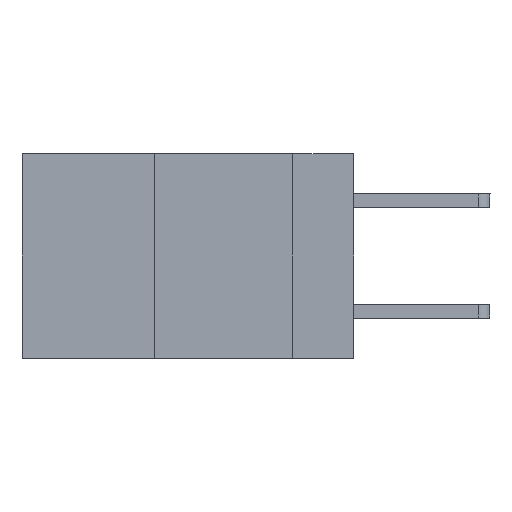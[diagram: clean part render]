
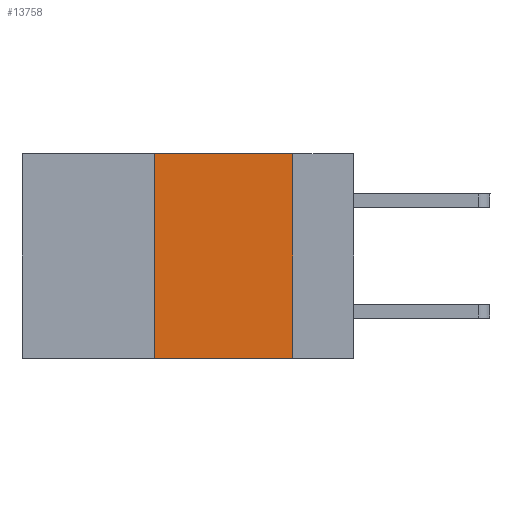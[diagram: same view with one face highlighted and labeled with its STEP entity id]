
A CAD part, left-side view. The second image highlights one B-rep face of the part: STEP entity #13758.
In plain terms, the highlighted planar face has unit normal (-1, 0, 0).
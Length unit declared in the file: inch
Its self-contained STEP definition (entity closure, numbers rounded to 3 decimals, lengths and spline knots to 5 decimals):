
#83 = CARTESIAN_POINT ( 'NONE',  ( 0., 0.11, 0. ) ) ;
#587 = VECTOR ( 'NONE', #10461, 39.37008 ) ;
#1218 = VECTOR ( 'NONE', #8216, 39.37008 ) ;
#1810 = DIRECTION ( 'NONE',  ( 0., 0., -1. ) ) ;
#2190 = VERTEX_POINT ( 'NONE', #6162 ) ;
#2627 = CARTESIAN_POINT ( 'NONE',  ( 0., 0.36, 0. ) ) ;
#2972 = CARTESIAN_POINT ( 'NONE',  ( 0., 0.6, -0.37 ) ) ;
#3174 = CARTESIAN_POINT ( 'NONE',  ( 0., 0.36, 0. ) ) ;
#3320 = ORIENTED_EDGE ( 'NONE', *, *, #9766, .F. ) ;
#3522 = CARTESIAN_POINT ( 'NONE',  ( 0., 0.11, 0. ) ) ;
#3816 = ORIENTED_EDGE ( 'NONE', *, *, #10767, .T. ) ;
#4796 = EDGE_CURVE ( 'NONE', #6194, #9662, #13932, .T. ) ;
#5835 = AXIS2_PLACEMENT_3D ( 'NONE', #10634, #9483, #1810 ) ;
#6048 = ORIENTED_EDGE ( 'NONE', *, *, #4796, .F. ) ;
#6162 = CARTESIAN_POINT ( 'NONE',  ( 0., 0.36, -0.37 ) ) ;
#6194 = VERTEX_POINT ( 'NONE', #83 ) ;
#6307 = DIRECTION ( 'NONE',  ( 0., 0., -1. ) ) ;
#7286 = FACE_OUTER_BOUND ( 'NONE', #12779, .T. ) ;
#7760 = VERTEX_POINT ( 'NONE', #3174 ) ;
#8181 = VECTOR ( 'NONE', #6307, 39.37008 ) ;
#8216 = DIRECTION ( 'NONE',  ( 0., -1., 0. ) ) ;
#8946 = VECTOR ( 'NONE', #12245, 39.37008 ) ;
#9180 = LINE ( 'NONE', #2972, #587 ) ;
#9276 = LINE ( 'NONE', #9348, #1218 ) ;
#9348 = CARTESIAN_POINT ( 'NONE',  ( 0., 0.6, 0. ) ) ;
#9483 = DIRECTION ( 'NONE',  ( 1., 0., 0. ) ) ;
#9662 = VERTEX_POINT ( 'NONE', #13334 ) ;
#9766 = EDGE_CURVE ( 'NONE', #7760, #6194, #9276, .T. ) ;
#10170 = ORIENTED_EDGE ( 'NONE', *, *, #12642, .F. ) ;
#10461 = DIRECTION ( 'NONE',  ( 0., -1., 0. ) ) ;
#10634 = CARTESIAN_POINT ( 'NONE',  ( 0., 0.6, 0. ) ) ;
#10767 = EDGE_CURVE ( 'NONE', #2190, #9662, #9180, .T. ) ;
#11617 = PLANE ( 'NONE',  #5835 ) ;
#11959 = LINE ( 'NONE', #2627, #8946 ) ;
#12245 = DIRECTION ( 'NONE',  ( 0., 0., 1. ) ) ;
#12642 = EDGE_CURVE ( 'NONE', #2190, #7760, #11959, .T. ) ;
#12779 = EDGE_LOOP ( 'NONE', ( #6048, #3320, #10170, #3816 ) ) ;
#13334 = CARTESIAN_POINT ( 'NONE',  ( 0., 0.11, -0.37 ) ) ;
#13758 = ADVANCED_FACE ( 'NONE', ( #7286 ), #11617, .F. ) ;
#13932 = LINE ( 'NONE', #3522, #8181 ) ;
